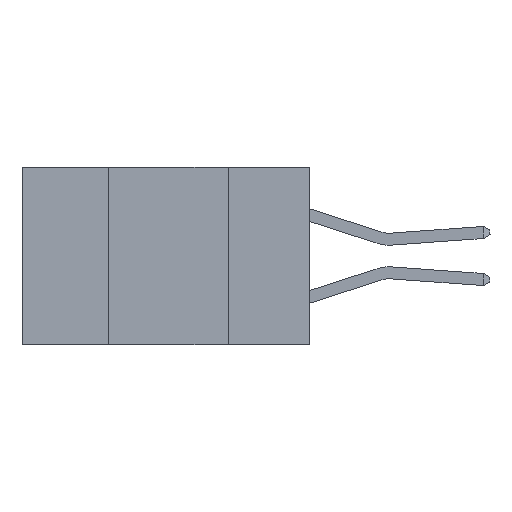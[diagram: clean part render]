
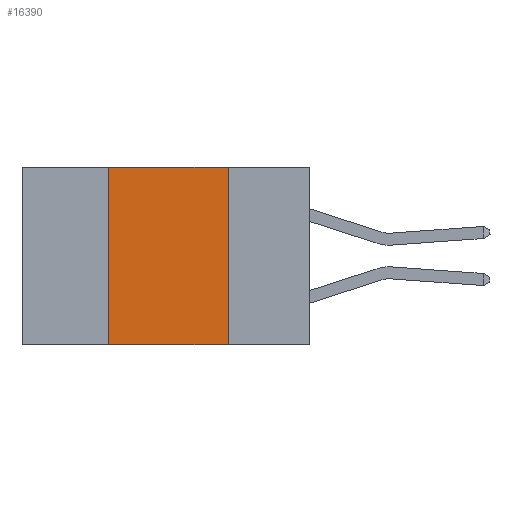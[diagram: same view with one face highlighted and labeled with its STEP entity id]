
A CAD part, left-side view. The second image highlights one B-rep face of the part: STEP entity #16390.
In plain terms, the highlighted planar face has unit normal (-1, 0, 0).
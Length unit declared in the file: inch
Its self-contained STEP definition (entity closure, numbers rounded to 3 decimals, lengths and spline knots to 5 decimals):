
#163 = CARTESIAN_POINT ( 'NONE',  ( 0., 0.42, -0.37 ) ) ;
#440 = CARTESIAN_POINT ( 'NONE',  ( 0., 0.6, 0. ) ) ;
#468 = ORIENTED_EDGE ( 'NONE', *, *, #6853, .F. ) ;
#930 = ORIENTED_EDGE ( 'NONE', *, *, #9254, .F. ) ;
#1400 = LINE ( 'NONE', #2466, #17573 ) ;
#2384 = VERTEX_POINT ( 'NONE', #163 ) ;
#2466 = CARTESIAN_POINT ( 'NONE',  ( 0., 0.42, -0.37 ) ) ;
#2879 = EDGE_CURVE ( 'NONE', #2384, #14667, #5553, .T. ) ;
#4425 = CARTESIAN_POINT ( 'NONE',  ( 0., 0.17, -0.37 ) ) ;
#4563 = ORIENTED_EDGE ( 'NONE', *, *, #12326, .F. ) ;
#5022 = VECTOR ( 'NONE', #13963, 39.37008 ) ;
#5443 = VERTEX_POINT ( 'NONE', #10165 ) ;
#5469 = DIRECTION ( 'NONE',  ( 0., -1., 0. ) ) ;
#5553 = LINE ( 'NONE', #11995, #6914 ) ;
#6494 = VERTEX_POINT ( 'NONE', #7217 ) ;
#6565 = CARTESIAN_POINT ( 'NONE',  ( 0., 0.6, 0. ) ) ;
#6853 = EDGE_CURVE ( 'NONE', #2384, #6494, #1400, .T. ) ;
#6914 = VECTOR ( 'NONE', #5469, 39.37008 ) ;
#7217 = CARTESIAN_POINT ( 'NONE',  ( 0., 0.42, 0. ) ) ;
#8168 = DIRECTION ( 'NONE',  ( 0., 0., -1. ) ) ;
#8532 = VECTOR ( 'NONE', #17070, 39.37008 ) ;
#9254 = EDGE_CURVE ( 'NONE', #5443, #14667, #15034, .T. ) ;
#10165 = CARTESIAN_POINT ( 'NONE',  ( 0., 0.17, 0. ) ) ;
#10668 = PLANE ( 'NONE',  #13045 ) ;
#11995 = CARTESIAN_POINT ( 'NONE',  ( 0., 0.6, -0.37 ) ) ;
#12326 = EDGE_CURVE ( 'NONE', #6494, #5443, #16803, .T. ) ;
#13045 = AXIS2_PLACEMENT_3D ( 'NONE', #6565, #14956, #8168 ) ;
#13723 = FACE_OUTER_BOUND ( 'NONE', #14414, .T. ) ;
#13963 = DIRECTION ( 'NONE',  ( 0., 0., -1. ) ) ;
#14414 = EDGE_LOOP ( 'NONE', ( #930, #4563, #468, #17137 ) ) ;
#14667 = VERTEX_POINT ( 'NONE', #4425 ) ;
#14941 = CARTESIAN_POINT ( 'NONE',  ( 0., 0.17, -0.37 ) ) ;
#14956 = DIRECTION ( 'NONE',  ( 1., 0., 0. ) ) ;
#15034 = LINE ( 'NONE', #14941, #5022 ) ;
#16324 = DIRECTION ( 'NONE',  ( 0., 0., 1. ) ) ;
#16390 = ADVANCED_FACE ( 'NONE', ( #13723 ), #10668, .F. ) ;
#16803 = LINE ( 'NONE', #440, #8532 ) ;
#17070 = DIRECTION ( 'NONE',  ( 0., -1., 0. ) ) ;
#17137 = ORIENTED_EDGE ( 'NONE', *, *, #2879, .T. ) ;
#17573 = VECTOR ( 'NONE', #16324, 39.37008 ) ;
